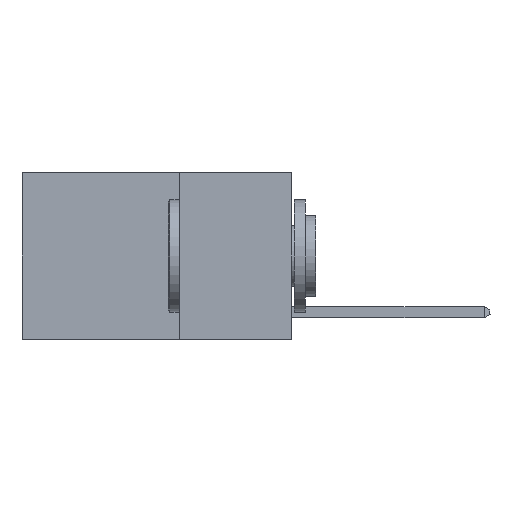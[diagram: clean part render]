
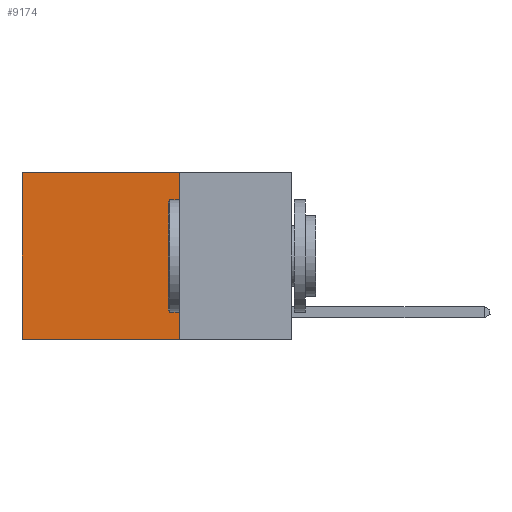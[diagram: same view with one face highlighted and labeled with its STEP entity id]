
A CAD part, left-side view. The second image highlights one B-rep face of the part: STEP entity #9174.
In plain terms, the highlighted planar face has unit normal (-1, 0, 0).
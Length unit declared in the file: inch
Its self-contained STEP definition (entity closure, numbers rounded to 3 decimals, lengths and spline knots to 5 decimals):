
#1925 = LINE ( 'NONE', #16695, #13628 ) ;
#2298 = VECTOR ( 'NONE', #16627, 39.37008 ) ;
#2932 = CARTESIAN_POINT ( 'NONE',  ( 0.2625, 0.6, -0.37 ) ) ;
#3133 = CARTESIAN_POINT ( 'NONE',  ( 0.2625, 0.25, 0. ) ) ;
#3477 = CARTESIAN_POINT ( 'NONE',  ( 0.2625, 0.25, 0. ) ) ;
#4000 = DIRECTION ( 'NONE',  ( 0., 0., -1. ) ) ;
#4738 = CARTESIAN_POINT ( 'NONE',  ( 0.2625, 0.25, 0. ) ) ;
#4993 = FACE_OUTER_BOUND ( 'NONE', #7454, .T. ) ;
#5407 = VERTEX_POINT ( 'NONE', #12247 ) ;
#5543 = EDGE_CURVE ( 'NONE', #12873, #5407, #23069, .T. ) ;
#5611 = EDGE_CURVE ( 'NONE', #12873, #20128, #12344, .T. ) ;
#6523 = ORIENTED_EDGE ( 'NONE', *, *, #21530, .F. ) ;
#7454 = EDGE_LOOP ( 'NONE', ( #13528, #6523, #23475, #22712 ) ) ;
#9174 = ADVANCED_FACE ( 'NONE', ( #4993 ), #14604, .F. ) ;
#9412 = DIRECTION ( 'NONE',  ( 0., 0., -1. ) ) ;
#10558 = DIRECTION ( 'NONE',  ( 1., 0., 0. ) ) ;
#10797 = LINE ( 'NONE', #23887, #12039 ) ;
#12025 = VERTEX_POINT ( 'NONE', #2932 ) ;
#12039 = VECTOR ( 'NONE', #20156, 39.37008 ) ;
#12247 = CARTESIAN_POINT ( 'NONE',  ( 0.2625, 0.25, -0.37 ) ) ;
#12344 = LINE ( 'NONE', #4738, #2298 ) ;
#12578 = AXIS2_PLACEMENT_3D ( 'NONE', #3477, #10558, #22301 ) ;
#12873 = VERTEX_POINT ( 'NONE', #3133 ) ;
#13528 = ORIENTED_EDGE ( 'NONE', *, *, #19838, .T. ) ;
#13628 = VECTOR ( 'NONE', #9412, 39.37008 ) ;
#14604 = PLANE ( 'NONE',  #12578 ) ;
#15855 = VECTOR ( 'NONE', #4000, 39.37008 ) ;
#16627 = DIRECTION ( 'NONE',  ( 0., 1., 0. ) ) ;
#16695 = CARTESIAN_POINT ( 'NONE',  ( 0.2625, 0.6, 0. ) ) ;
#17546 = CARTESIAN_POINT ( 'NONE',  ( 0.2625, 0.6, 0. ) ) ;
#18808 = CARTESIAN_POINT ( 'NONE',  ( 0.2625, 0.25, 0. ) ) ;
#19838 = EDGE_CURVE ( 'NONE', #20128, #12025, #1925, .T. ) ;
#20128 = VERTEX_POINT ( 'NONE', #17546 ) ;
#20156 = DIRECTION ( 'NONE',  ( 0., 1., 0. ) ) ;
#21530 = EDGE_CURVE ( 'NONE', #5407, #12025, #10797, .T. ) ;
#22301 = DIRECTION ( 'NONE',  ( 0., 0., -1. ) ) ;
#22712 = ORIENTED_EDGE ( 'NONE', *, *, #5611, .T. ) ;
#23069 = LINE ( 'NONE', #18808, #15855 ) ;
#23475 = ORIENTED_EDGE ( 'NONE', *, *, #5543, .F. ) ;
#23887 = CARTESIAN_POINT ( 'NONE',  ( 0.2625, 0.25, -0.37 ) ) ;
